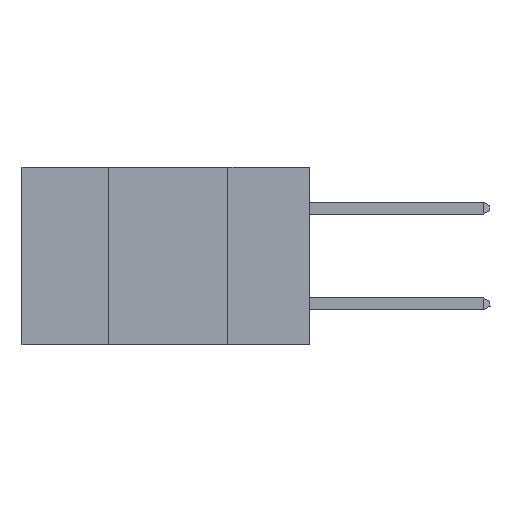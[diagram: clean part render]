
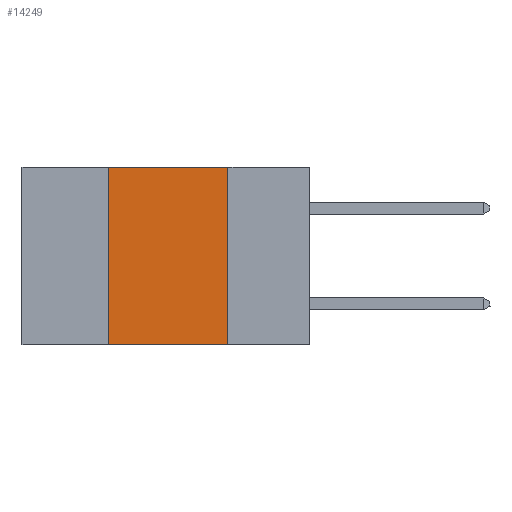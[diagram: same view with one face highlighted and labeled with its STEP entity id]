
A CAD part, left-side view. The second image highlights one B-rep face of the part: STEP entity #14249.
In plain terms, the highlighted planar face has unit normal (-1, 0, 0).
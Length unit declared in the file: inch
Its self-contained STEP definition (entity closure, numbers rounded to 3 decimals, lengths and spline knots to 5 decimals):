
#2476 = CARTESIAN_POINT ( 'NONE',  ( 0., 0.6, 0. ) ) ;
#2698 = FACE_OUTER_BOUND ( 'NONE', #8551, .T. ) ;
#3323 = EDGE_CURVE ( 'NONE', #17196, #16102, #16042, .T. ) ;
#4312 = CARTESIAN_POINT ( 'NONE',  ( 0., 0.6, -0.37 ) ) ;
#4793 = CARTESIAN_POINT ( 'NONE',  ( 0., 0.17, 0. ) ) ;
#4815 = EDGE_CURVE ( 'NONE', #9759, #9998, #13572, .T. ) ;
#5039 = VECTOR ( 'NONE', #7154, 39.37008 ) ;
#5240 = VECTOR ( 'NONE', #9934, 39.37008 ) ;
#5759 = CARTESIAN_POINT ( 'NONE',  ( 0., 0.42, 0. ) ) ;
#6143 = CARTESIAN_POINT ( 'NONE',  ( 0., 0.17, 0. ) ) ;
#6511 = VECTOR ( 'NONE', #16193, 39.37008 ) ;
#6719 = DIRECTION ( 'NONE',  ( 1., 0., 0. ) ) ;
#7059 = EDGE_CURVE ( 'NONE', #17196, #9759, #10751, .T. ) ;
#7154 = DIRECTION ( 'NONE',  ( 0., -1., 0. ) ) ;
#7636 = DIRECTION ( 'NONE',  ( 0., 0., -1. ) ) ;
#8125 = PLANE ( 'NONE',  #11644 ) ;
#8551 = EDGE_LOOP ( 'NONE', ( #15114, #15937, #13031, #15444 ) ) ;
#9759 = VERTEX_POINT ( 'NONE', #5759 ) ;
#9934 = DIRECTION ( 'NONE',  ( 0., -1., 0. ) ) ;
#9938 = CARTESIAN_POINT ( 'NONE',  ( 0., 0.17, -0.37 ) ) ;
#9949 = EDGE_CURVE ( 'NONE', #9998, #16102, #12455, .T. ) ;
#9998 = VERTEX_POINT ( 'NONE', #4793 ) ;
#10751 = LINE ( 'NONE', #14779, #6511 ) ;
#11644 = AXIS2_PLACEMENT_3D ( 'NONE', #2476, #6719, #16296 ) ;
#12255 = CARTESIAN_POINT ( 'NONE',  ( 0., 0.42, -0.37 ) ) ;
#12455 = LINE ( 'NONE', #6143, #15986 ) ;
#13031 = ORIENTED_EDGE ( 'NONE', *, *, #7059, .F. ) ;
#13572 = LINE ( 'NONE', #16570, #5240 ) ;
#14249 = ADVANCED_FACE ( 'NONE', ( #2698 ), #8125, .F. ) ;
#14779 = CARTESIAN_POINT ( 'NONE',  ( 0., 0.42, 0. ) ) ;
#15114 = ORIENTED_EDGE ( 'NONE', *, *, #9949, .F. ) ;
#15444 = ORIENTED_EDGE ( 'NONE', *, *, #3323, .T. ) ;
#15937 = ORIENTED_EDGE ( 'NONE', *, *, #4815, .F. ) ;
#15986 = VECTOR ( 'NONE', #7636, 39.37008 ) ;
#16042 = LINE ( 'NONE', #4312, #5039 ) ;
#16102 = VERTEX_POINT ( 'NONE', #9938 ) ;
#16193 = DIRECTION ( 'NONE',  ( 0., 0., 1. ) ) ;
#16296 = DIRECTION ( 'NONE',  ( 0., 0., -1. ) ) ;
#16570 = CARTESIAN_POINT ( 'NONE',  ( 0., 0.6, 0. ) ) ;
#17196 = VERTEX_POINT ( 'NONE', #12255 ) ;
